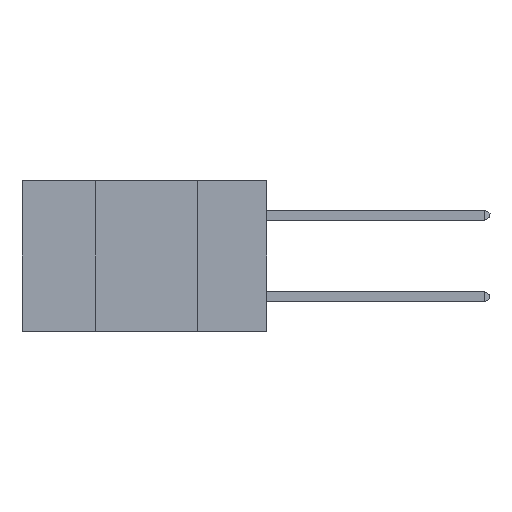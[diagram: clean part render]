
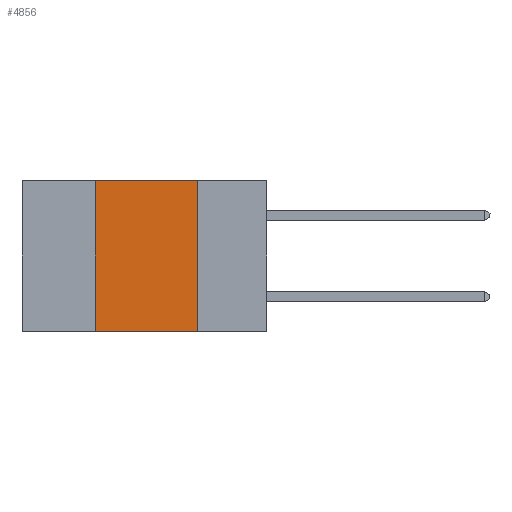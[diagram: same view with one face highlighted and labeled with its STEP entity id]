
A CAD part, left-side view. The second image highlights one B-rep face of the part: STEP entity #4856.
In plain terms, the highlighted planar face has unit normal (-1, 0, 0).
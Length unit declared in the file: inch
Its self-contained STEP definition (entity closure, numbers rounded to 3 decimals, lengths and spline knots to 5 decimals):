
#174 = LINE ( 'NONE', #2523, #13264 ) ;
#653 = CARTESIAN_POINT ( 'NONE',  ( 0., 0.42, -0.37 ) ) ;
#732 = DIRECTION ( 'NONE',  ( 1., 0., 0. ) ) ;
#910 = EDGE_CURVE ( 'NONE', #13868, #1754, #3041, .T. ) ;
#1430 = ORIENTED_EDGE ( 'NONE', *, *, #910, .F. ) ;
#1752 = CARTESIAN_POINT ( 'NONE',  ( 0., 0.6, -0.37 ) ) ;
#1754 = VERTEX_POINT ( 'NONE', #7888 ) ;
#2523 = CARTESIAN_POINT ( 'NONE',  ( 0., 0.42, 0. ) ) ;
#3041 = LINE ( 'NONE', #6927, #14935 ) ;
#3354 = ORIENTED_EDGE ( 'NONE', *, *, #15612, .F. ) ;
#3668 = VERTEX_POINT ( 'NONE', #653 ) ;
#3801 = CARTESIAN_POINT ( 'NONE',  ( 0., 0.17, -0.37 ) ) ;
#4781 = ORIENTED_EDGE ( 'NONE', *, *, #15248, .F. ) ;
#4856 = ADVANCED_FACE ( 'NONE', ( #9764 ), #15682, .F. ) ;
#5729 = VERTEX_POINT ( 'NONE', #3801 ) ;
#5809 = VECTOR ( 'NONE', #6861, 39.37008 ) ;
#6861 = DIRECTION ( 'NONE',  ( 0., -1., 0. ) ) ;
#6927 = CARTESIAN_POINT ( 'NONE',  ( 0., 0.6, 0. ) ) ;
#7250 = CARTESIAN_POINT ( 'NONE',  ( 0., 0.6, 0. ) ) ;
#7888 = CARTESIAN_POINT ( 'NONE',  ( 0., 0.17, 0. ) ) ;
#9092 = VECTOR ( 'NONE', #14269, 39.37008 ) ;
#9491 = LINE ( 'NONE', #1752, #5809 ) ;
#9718 = DIRECTION ( 'NONE',  ( 0., 0., -1. ) ) ;
#9764 = FACE_OUTER_BOUND ( 'NONE', #15303, .T. ) ;
#10316 = ORIENTED_EDGE ( 'NONE', *, *, #15563, .T. ) ;
#11561 = LINE ( 'NONE', #15417, #9092 ) ;
#12021 = CARTESIAN_POINT ( 'NONE',  ( 0., 0.42, 0. ) ) ;
#13264 = VECTOR ( 'NONE', #16051, 39.37008 ) ;
#13868 = VERTEX_POINT ( 'NONE', #12021 ) ;
#14269 = DIRECTION ( 'NONE',  ( 0., 0., -1. ) ) ;
#14935 = VECTOR ( 'NONE', #15021, 39.37008 ) ;
#15021 = DIRECTION ( 'NONE',  ( 0., -1., 0. ) ) ;
#15248 = EDGE_CURVE ( 'NONE', #3668, #13868, #174, .T. ) ;
#15303 = EDGE_LOOP ( 'NONE', ( #3354, #1430, #4781, #10316 ) ) ;
#15417 = CARTESIAN_POINT ( 'NONE',  ( 0., 0.17, 0. ) ) ;
#15563 = EDGE_CURVE ( 'NONE', #3668, #5729, #9491, .T. ) ;
#15612 = EDGE_CURVE ( 'NONE', #1754, #5729, #11561, .T. ) ;
#15654 = AXIS2_PLACEMENT_3D ( 'NONE', #7250, #732, #9718 ) ;
#15682 = PLANE ( 'NONE',  #15654 ) ;
#16051 = DIRECTION ( 'NONE',  ( 0., 0., 1. ) ) ;
